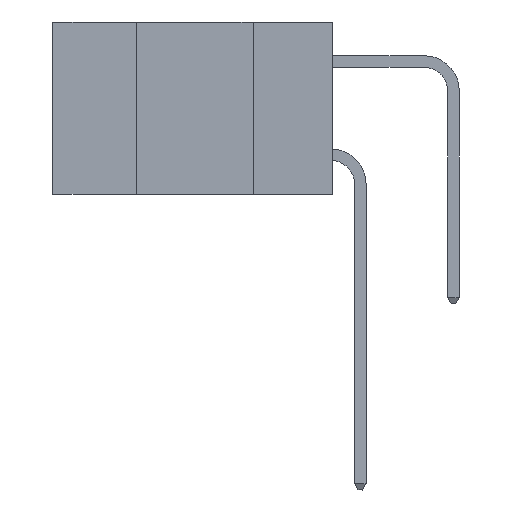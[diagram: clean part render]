
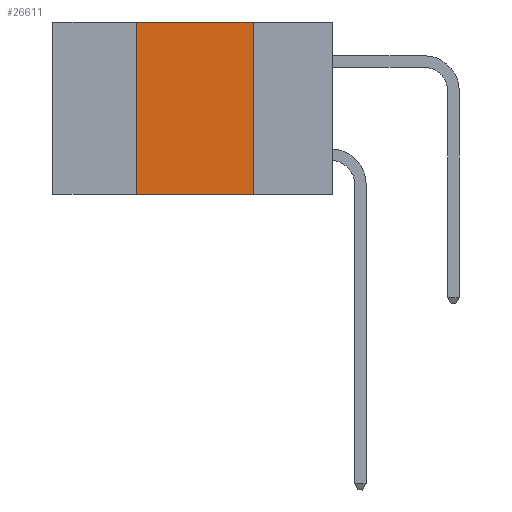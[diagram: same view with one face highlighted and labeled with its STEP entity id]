
A CAD part, left-side view. The second image highlights one B-rep face of the part: STEP entity #26611.
In plain terms, the highlighted planar face has unit normal (-1, 0, 0).
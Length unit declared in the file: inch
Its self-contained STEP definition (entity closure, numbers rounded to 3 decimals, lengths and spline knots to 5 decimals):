
#2292 = LINE ( 'NONE', #3813, #9502 ) ;
#3275 = DIRECTION ( 'NONE',  ( 0., -1., 0. ) ) ;
#3813 = CARTESIAN_POINT ( 'NONE',  ( 0., 0.42, 0. ) ) ;
#4134 = AXIS2_PLACEMENT_3D ( 'NONE', #27431, #30149, #13906 ) ;
#4416 = DIRECTION ( 'NONE',  ( 0., -1., 0. ) ) ;
#5901 = ORIENTED_EDGE ( 'NONE', *, *, #23789, .T. ) ;
#6910 = LINE ( 'NONE', #30138, #27741 ) ;
#8856 = ORIENTED_EDGE ( 'NONE', *, *, #31695, .F. ) ;
#9502 = VECTOR ( 'NONE', #20148, 39.37008 ) ;
#10272 = VECTOR ( 'NONE', #4416, 39.37008 ) ;
#11191 = PLANE ( 'NONE',  #4134 ) ;
#12919 = CARTESIAN_POINT ( 'NONE',  ( 0., 0.42, -0.37 ) ) ;
#13530 = VERTEX_POINT ( 'NONE', #12919 ) ;
#13906 = DIRECTION ( 'NONE',  ( 0., 0., -1. ) ) ;
#14000 = DIRECTION ( 'NONE',  ( 0., 0., -1. ) ) ;
#14896 = CARTESIAN_POINT ( 'NONE',  ( 0., 0.6, 0. ) ) ;
#16839 = CARTESIAN_POINT ( 'NONE',  ( 0., 0.6, -0.37 ) ) ;
#16924 = VERTEX_POINT ( 'NONE', #29685 ) ;
#17527 = LINE ( 'NONE', #14896, #10272 ) ;
#17852 = ORIENTED_EDGE ( 'NONE', *, *, #22588, .F. ) ;
#20021 = FACE_OUTER_BOUND ( 'NONE', #34973, .T. ) ;
#20148 = DIRECTION ( 'NONE',  ( 0., 0., 1. ) ) ;
#22588 = EDGE_CURVE ( 'NONE', #13530, #28243, #2292, .T. ) ;
#23099 = EDGE_CURVE ( 'NONE', #31256, #16924, #6910, .T. ) ;
#23789 = EDGE_CURVE ( 'NONE', #13530, #16924, #24427, .T. ) ;
#24283 = CARTESIAN_POINT ( 'NONE',  ( 0., 0.17, 0. ) ) ;
#24427 = LINE ( 'NONE', #16839, #30763 ) ;
#25666 = CARTESIAN_POINT ( 'NONE',  ( 0., 0.42, 0. ) ) ;
#26319 = ORIENTED_EDGE ( 'NONE', *, *, #23099, .F. ) ;
#26611 = ADVANCED_FACE ( 'NONE', ( #20021 ), #11191, .F. ) ;
#27431 = CARTESIAN_POINT ( 'NONE',  ( 0., 0.6, 0. ) ) ;
#27741 = VECTOR ( 'NONE', #14000, 39.37008 ) ;
#28243 = VERTEX_POINT ( 'NONE', #25666 ) ;
#29685 = CARTESIAN_POINT ( 'NONE',  ( 0., 0.17, -0.37 ) ) ;
#30138 = CARTESIAN_POINT ( 'NONE',  ( 0., 0.17, 0. ) ) ;
#30149 = DIRECTION ( 'NONE',  ( 1., 0., 0. ) ) ;
#30763 = VECTOR ( 'NONE', #3275, 39.37008 ) ;
#31256 = VERTEX_POINT ( 'NONE', #24283 ) ;
#31695 = EDGE_CURVE ( 'NONE', #28243, #31256, #17527, .T. ) ;
#34973 = EDGE_LOOP ( 'NONE', ( #26319, #8856, #17852, #5901 ) ) ;
